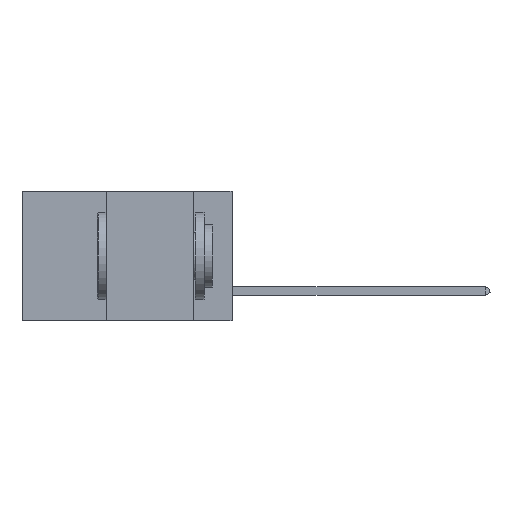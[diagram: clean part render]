
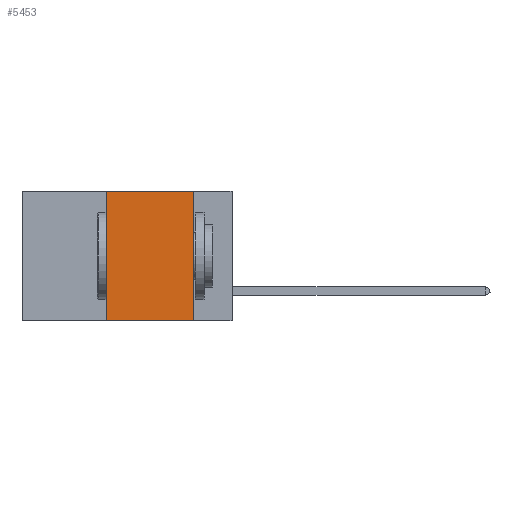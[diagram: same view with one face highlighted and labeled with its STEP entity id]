
A CAD part, left-side view. The second image highlights one B-rep face of the part: STEP entity #5453.
In plain terms, the highlighted planar face has unit normal (-1, 0, 0).
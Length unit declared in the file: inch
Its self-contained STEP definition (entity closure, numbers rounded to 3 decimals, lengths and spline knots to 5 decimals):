
#62 = CARTESIAN_POINT ( 'NONE',  ( 0., 0.11, -0.37 ) ) ;
#78 = EDGE_CURVE ( 'NONE', #18750, #4254, #11869, .T. ) ;
#1031 = DIRECTION ( 'NONE',  ( 0., 0., 1. ) ) ;
#1097 = EDGE_CURVE ( 'NONE', #4254, #7766, #12388, .T. ) ;
#4254 = VERTEX_POINT ( 'NONE', #17594 ) ;
#4836 = ORIENTED_EDGE ( 'NONE', *, *, #78, .F. ) ;
#5100 = EDGE_CURVE ( 'NONE', #7766, #6088, #9574, .T. ) ;
#5361 = VECTOR ( 'NONE', #10055, 39.37008 ) ;
#5453 = ADVANCED_FACE ( 'NONE', ( #19886 ), #15403, .F. ) ;
#5872 = LINE ( 'NONE', #17040, #18456 ) ;
#5994 = EDGE_CURVE ( 'NONE', #18750, #6088, #5872, .T. ) ;
#6088 = VERTEX_POINT ( 'NONE', #62 ) ;
#6315 = ORIENTED_EDGE ( 'NONE', *, *, #5100, .F. ) ;
#6805 = CARTESIAN_POINT ( 'NONE',  ( 0., 0.11, 0. ) ) ;
#7766 = VERTEX_POINT ( 'NONE', #6805 ) ;
#7900 = VECTOR ( 'NONE', #10714, 39.37008 ) ;
#8089 = DIRECTION ( 'NONE',  ( 1., 0., 0. ) ) ;
#9574 = LINE ( 'NONE', #12725, #7900 ) ;
#10055 = DIRECTION ( 'NONE',  ( 0., -1., 0. ) ) ;
#10714 = DIRECTION ( 'NONE',  ( 0., 0., -1. ) ) ;
#11082 = CARTESIAN_POINT ( 'NONE',  ( 0., 0.36, -0.37 ) ) ;
#11869 = LINE ( 'NONE', #14659, #17730 ) ;
#12388 = LINE ( 'NONE', #18947, #5361 ) ;
#12725 = CARTESIAN_POINT ( 'NONE',  ( 0., 0.11, 0. ) ) ;
#13520 = DIRECTION ( 'NONE',  ( 0., 0., -1. ) ) ;
#14063 = AXIS2_PLACEMENT_3D ( 'NONE', #17025, #8089, #13520 ) ;
#14659 = CARTESIAN_POINT ( 'NONE',  ( 0., 0.36, 0. ) ) ;
#15403 = PLANE ( 'NONE',  #14063 ) ;
#17025 = CARTESIAN_POINT ( 'NONE',  ( 0., 0.6, 0. ) ) ;
#17040 = CARTESIAN_POINT ( 'NONE',  ( 0., 0.6, -0.37 ) ) ;
#17346 = ORIENTED_EDGE ( 'NONE', *, *, #1097, .F. ) ;
#17594 = CARTESIAN_POINT ( 'NONE',  ( 0., 0.36, 0. ) ) ;
#17730 = VECTOR ( 'NONE', #1031, 39.37008 ) ;
#18456 = VECTOR ( 'NONE', #18856, 39.37008 ) ;
#18750 = VERTEX_POINT ( 'NONE', #11082 ) ;
#18856 = DIRECTION ( 'NONE',  ( 0., -1., 0. ) ) ;
#18947 = CARTESIAN_POINT ( 'NONE',  ( 0., 0.6, 0. ) ) ;
#19886 = FACE_OUTER_BOUND ( 'NONE', #20100, .T. ) ;
#20100 = EDGE_LOOP ( 'NONE', ( #6315, #17346, #4836, #22788 ) ) ;
#22788 = ORIENTED_EDGE ( 'NONE', *, *, #5994, .T. ) ;
